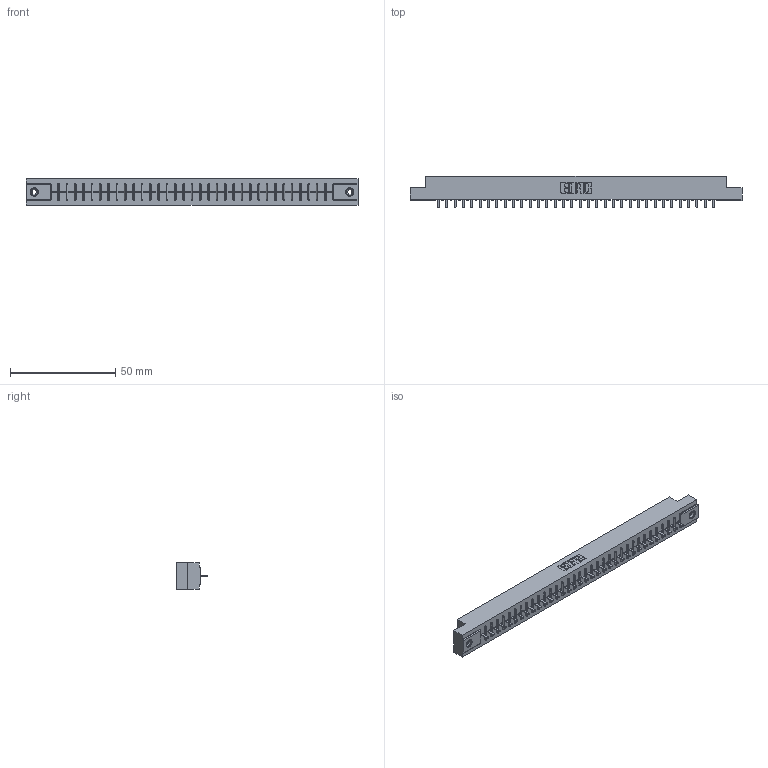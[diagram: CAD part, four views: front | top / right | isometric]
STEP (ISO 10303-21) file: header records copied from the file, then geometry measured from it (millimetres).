
FILE_DESCRIPTION (( 'STEP AP203' ), '1' );
FILE_NAME ('306-034-421-108.STEP', '2020-09-22T03:32:28', ( '' ), ( '' ), 'SwSTEP 2.0', 'SolidWorks 2020', '' );
FILE_SCHEMA (( 'CONFIG_CONTROL_DESIGN' ));
Length unit declared in the file: inch
Products named in the file (4): 345-250-001_345-250-003-102; 306 Part_.156 Dia; 306-290-001_121; 306-034-421-108
Assembly tree (37 placements, depth 2):
  306-034-421-108
    306 Part_.156 Dia
    306-290-001_121  x34
    345-250-001_345-250-003-102  x2
Bounding box: 157.73 x 14.88 x 12.7 mm (x, y, z)
Volume: 17318.5 mm3; surface area: 17468.7 mm2
Topology: 37 solids, 37 shells, 2556 faces, 7150 edges, 4576 vertices
Faces by surface type: plane 1698, cylinder 706, sphere 136, cone 12, torus 4
Entity records: 33884 total; most frequent: CARTESIAN_POINT 5668, ORIENTED_EDGE 5612, DIRECTION 5598, EDGE_CURVE 2806, VECTOR 2190, LINE 2190, VERTEX_POINT 1774, AXIS2_PLACEMENT_3D 1704
